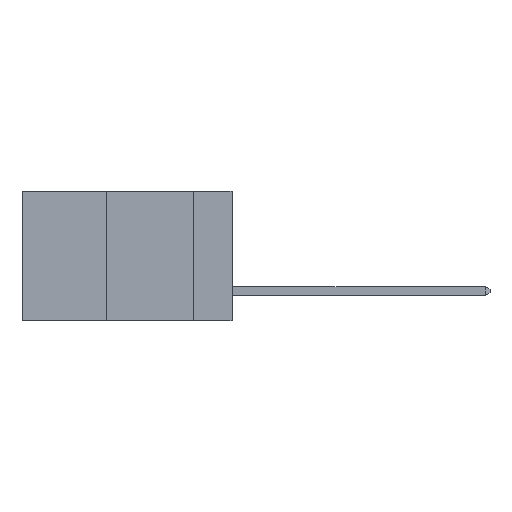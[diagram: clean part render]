
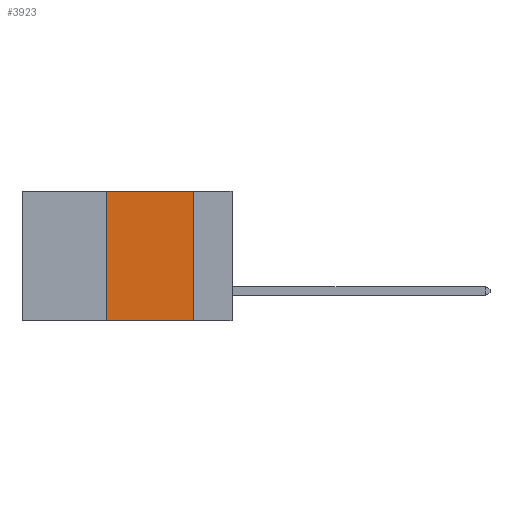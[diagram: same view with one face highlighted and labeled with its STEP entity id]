
A CAD part, left-side view. The second image highlights one B-rep face of the part: STEP entity #3923.
In plain terms, the highlighted planar face has unit normal (-1, 0, 0).
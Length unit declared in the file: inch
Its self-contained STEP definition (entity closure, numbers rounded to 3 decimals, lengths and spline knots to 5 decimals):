
#127 = EDGE_CURVE ( 'NONE', #7751, #4713, #6262, .T. ) ;
#503 = LINE ( 'NONE', #1087, #3124 ) ;
#620 = CARTESIAN_POINT ( 'NONE',  ( 0., 0.11, -0.37 ) ) ;
#992 = ORIENTED_EDGE ( 'NONE', *, *, #9912, .F. ) ;
#1087 = CARTESIAN_POINT ( 'NONE',  ( 0., 0.11, 0. ) ) ;
#1613 = ORIENTED_EDGE ( 'NONE', *, *, #9293, .F. ) ;
#1734 = ORIENTED_EDGE ( 'NONE', *, *, #9884, .F. ) ;
#1742 = AXIS2_PLACEMENT_3D ( 'NONE', #6791, #6834, #6822 ) ;
#2146 = ORIENTED_EDGE ( 'NONE', *, *, #127, .T. ) ;
#2147 = DIRECTION ( 'NONE',  ( 0., 0., 1. ) ) ;
#2173 = VECTOR ( 'NONE', #5481, 39.37008 ) ;
#2474 = LINE ( 'NONE', #6220, #4232 ) ;
#2877 = VECTOR ( 'NONE', #5325, 39.37008 ) ;
#3106 = VERTEX_POINT ( 'NONE', #4921 ) ;
#3124 = VECTOR ( 'NONE', #6065, 39.37008 ) ;
#3923 = ADVANCED_FACE ( 'NONE', ( #4223 ), #6857, .F. ) ;
#4223 = FACE_OUTER_BOUND ( 'NONE', #4715, .T. ) ;
#4232 = VECTOR ( 'NONE', #2147, 39.37008 ) ;
#4523 = CARTESIAN_POINT ( 'NONE',  ( 0., 0.6, 0. ) ) ;
#4713 = VERTEX_POINT ( 'NONE', #620 ) ;
#4715 = EDGE_LOOP ( 'NONE', ( #992, #1734, #1613, #2146 ) ) ;
#4921 = CARTESIAN_POINT ( 'NONE',  ( 0., 0.11, 0. ) ) ;
#5325 = DIRECTION ( 'NONE',  ( 0., -1., 0. ) ) ;
#5481 = DIRECTION ( 'NONE',  ( 0., -1., 0. ) ) ;
#5502 = CARTESIAN_POINT ( 'NONE',  ( 0., 0.6, -0.37 ) ) ;
#6065 = DIRECTION ( 'NONE',  ( 0., 0., -1. ) ) ;
#6220 = CARTESIAN_POINT ( 'NONE',  ( 0., 0.36, 0. ) ) ;
#6262 = LINE ( 'NONE', #5502, #2173 ) ;
#6791 = CARTESIAN_POINT ( 'NONE',  ( 0., 0.6, 0. ) ) ;
#6822 = DIRECTION ( 'NONE',  ( 0., 0., -1. ) ) ;
#6834 = DIRECTION ( 'NONE',  ( 1., 0., 0. ) ) ;
#6857 = PLANE ( 'NONE',  #1742 ) ;
#7422 = VERTEX_POINT ( 'NONE', #9904 ) ;
#7629 = CARTESIAN_POINT ( 'NONE',  ( 0., 0.36, -0.37 ) ) ;
#7751 = VERTEX_POINT ( 'NONE', #7629 ) ;
#8815 = LINE ( 'NONE', #4523, #2877 ) ;
#9293 = EDGE_CURVE ( 'NONE', #7751, #7422, #2474, .T. ) ;
#9884 = EDGE_CURVE ( 'NONE', #7422, #3106, #8815, .T. ) ;
#9904 = CARTESIAN_POINT ( 'NONE',  ( 0., 0.36, 0. ) ) ;
#9912 = EDGE_CURVE ( 'NONE', #3106, #4713, #503, .T. ) ;
